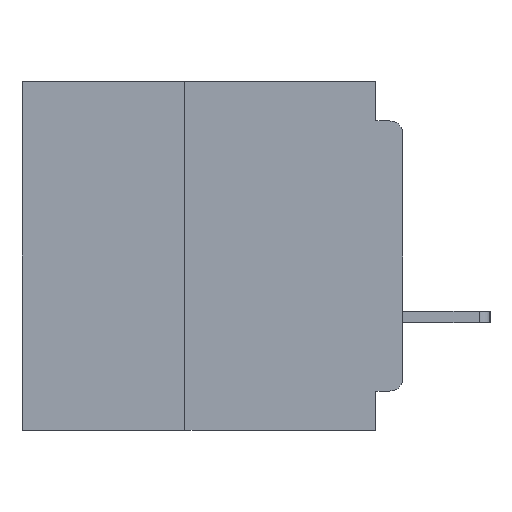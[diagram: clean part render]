
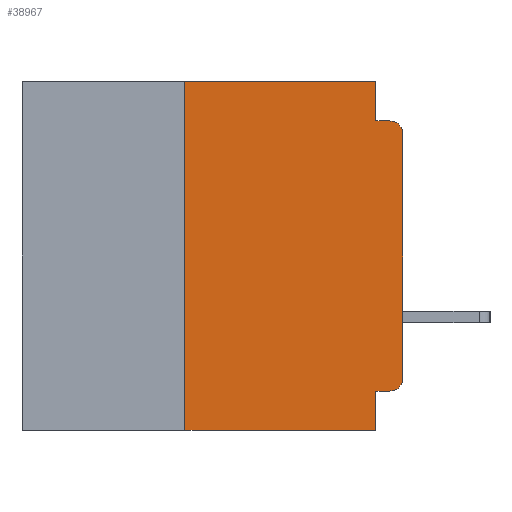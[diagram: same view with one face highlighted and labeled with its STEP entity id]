
A CAD part, left-side view. The second image highlights one B-rep face of the part: STEP entity #38967.
In plain terms, the highlighted planar face has unit normal (-1, 0, 0).
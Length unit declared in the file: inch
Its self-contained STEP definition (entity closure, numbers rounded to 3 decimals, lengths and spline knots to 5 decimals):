
#1255 = VERTEX_POINT ( 'NONE', #56523 ) ;
#1685 = EDGE_CURVE ( 'NONE', #65093, #3620, #50024, .T. ) ;
#2430 = CARTESIAN_POINT ( 'NONE',  ( 0., 0.015, -0.355 ) ) ;
#2866 = VECTOR ( 'NONE', #17412, 39.37008 ) ;
#3620 = VERTEX_POINT ( 'NONE', #35172 ) ;
#4160 = PLANE ( 'NONE',  #16183 ) ;
#7343 = CARTESIAN_POINT ( 'NONE',  ( 0., 0.031, 0. ) ) ;
#7485 = CARTESIAN_POINT ( 'NONE',  ( 0., 0.015, -0.34 ) ) ;
#7657 = LINE ( 'NONE', #48281, #29862 ) ;
#7855 = DIRECTION ( 'NONE',  ( 0., 0., 1. ) ) ;
#8508 = EDGE_CURVE ( 'NONE', #1255, #65093, #61952, .T. ) ;
#9325 = ORIENTED_EDGE ( 'NONE', *, *, #62804, .F. ) ;
#10684 = EDGE_LOOP ( 'NONE', ( #64152, #30747, #50176, #18854, #46270, #9325, #41486, #35100, #15360, #61409 ) ) ;
#12639 = DIRECTION ( 'NONE',  ( 0., 0., -1. ) ) ;
#14378 = DIRECTION ( 'NONE',  ( 1., 0., 0. ) ) ;
#14414 = VECTOR ( 'NONE', #64098, 39.37008 ) ;
#15226 = VECTOR ( 'NONE', #37704, 39.37008 ) ;
#15360 = ORIENTED_EDGE ( 'NONE', *, *, #49907, .F. ) ;
#16049 = EDGE_CURVE ( 'NONE', #16051, #1255, #30943, .T. ) ;
#16051 = VERTEX_POINT ( 'NONE', #2430 ) ;
#16183 = AXIS2_PLACEMENT_3D ( 'NONE', #34315, #14378, #49643 ) ;
#16608 = CARTESIAN_POINT ( 'NONE',  ( 0., 0., 0. ) ) ;
#16840 = LINE ( 'NONE', #7343, #15226 ) ;
#17412 = DIRECTION ( 'NONE',  ( 0., 0., -1. ) ) ;
#18854 = ORIENTED_EDGE ( 'NONE', *, *, #26511, .F. ) ;
#20239 = VECTOR ( 'NONE', #26630, 39.37008 ) ;
#20734 = DIRECTION ( 'NONE',  ( 0., -1., 0. ) ) ;
#21391 = EDGE_CURVE ( 'NONE', #46968, #26798, #23236, .T. ) ;
#21931 = AXIS2_PLACEMENT_3D ( 'NONE', #43266, #43131, #43058 ) ;
#23236 = LINE ( 'NONE', #50883, #36675 ) ;
#25878 = CARTESIAN_POINT ( 'NONE',  ( 0., 0.25, 0. ) ) ;
#26257 = VECTOR ( 'NONE', #27592, 39.37008 ) ;
#26511 = EDGE_CURVE ( 'NONE', #58493, #40507, #16840, .T. ) ;
#26630 = DIRECTION ( 'NONE',  ( 0., -1., 0. ) ) ;
#26798 = VERTEX_POINT ( 'NONE', #64729 ) ;
#27592 = DIRECTION ( 'NONE',  ( 0., 1., 0. ) ) ;
#27931 = LINE ( 'NONE', #29056, #14414 ) ;
#29056 = CARTESIAN_POINT ( 'NONE',  ( 0., 0., -0.045 ) ) ;
#29128 = VERTEX_POINT ( 'NONE', #36117 ) ;
#29835 = LINE ( 'NONE', #47358, #2866 ) ;
#29862 = VECTOR ( 'NONE', #7855, 39.37008 ) ;
#30747 = ORIENTED_EDGE ( 'NONE', *, *, #1685, .T. ) ;
#30943 = CIRCLE ( 'NONE', #55826, 0.015 ) ;
#31742 = CARTESIAN_POINT ( 'NONE',  ( 0., 0.437, 0. ) ) ;
#32212 = VECTOR ( 'NONE', #41752, 39.37008 ) ;
#33148 = CARTESIAN_POINT ( 'NONE',  ( 0., 0.25, -0.4 ) ) ;
#34315 = CARTESIAN_POINT ( 'NONE',  ( 0., 0.437, 0. ) ) ;
#35100 = ORIENTED_EDGE ( 'NONE', *, *, #44341, .F. ) ;
#35172 = CARTESIAN_POINT ( 'NONE',  ( 0., 0.015, -0.045 ) ) ;
#35285 = LINE ( 'NONE', #31742, #20239 ) ;
#36117 = CARTESIAN_POINT ( 'NONE',  ( 0., 0.031, -0.355 ) ) ;
#36675 = VECTOR ( 'NONE', #20734, 39.37008 ) ;
#37704 = DIRECTION ( 'NONE',  ( 0., 0., -1. ) ) ;
#38109 = CARTESIAN_POINT ( 'NONE',  ( 0., 0.031, -0.045 ) ) ;
#38646 = EDGE_CURVE ( 'NONE', #43870, #58493, #35285, .T. ) ;
#38967 = ADVANCED_FACE ( 'NONE', ( #41519 ), #4160, .F. ) ;
#39283 = CARTESIAN_POINT ( 'NONE',  ( 0., 0.031, 0. ) ) ;
#40507 = VERTEX_POINT ( 'NONE', #38109 ) ;
#41486 = ORIENTED_EDGE ( 'NONE', *, *, #21391, .T. ) ;
#41519 = FACE_OUTER_BOUND ( 'NONE', #10684, .T. ) ;
#41752 = DIRECTION ( 'NONE',  ( 0., 0., 1. ) ) ;
#42884 = DIRECTION ( 'NONE',  ( -1., 0., 0. ) ) ;
#43058 = DIRECTION ( 'NONE',  ( 0., 0., -1. ) ) ;
#43131 = DIRECTION ( 'NONE',  ( -1., 0., 0. ) ) ;
#43182 = CARTESIAN_POINT ( 'NONE',  ( 0., 0., -0.06 ) ) ;
#43266 = CARTESIAN_POINT ( 'NONE',  ( 0., 0.015, -0.06 ) ) ;
#43870 = VERTEX_POINT ( 'NONE', #25878 ) ;
#44341 = EDGE_CURVE ( 'NONE', #29128, #26798, #29835, .T. ) ;
#46270 = ORIENTED_EDGE ( 'NONE', *, *, #38646, .F. ) ;
#46968 = VERTEX_POINT ( 'NONE', #33148 ) ;
#47358 = CARTESIAN_POINT ( 'NONE',  ( 0., 0.031, -0.4 ) ) ;
#48281 = CARTESIAN_POINT ( 'NONE',  ( 0., 0.25, -0.4 ) ) ;
#49486 = EDGE_CURVE ( 'NONE', #40507, #3620, #27931, .T. ) ;
#49643 = DIRECTION ( 'NONE',  ( 0., 0., -1. ) ) ;
#49907 = EDGE_CURVE ( 'NONE', #16051, #29128, #54577, .T. ) ;
#50024 = CIRCLE ( 'NONE', #21931, 0.015 ) ;
#50176 = ORIENTED_EDGE ( 'NONE', *, *, #49486, .F. ) ;
#50883 = CARTESIAN_POINT ( 'NONE',  ( 0., 0.437, -0.4 ) ) ;
#52625 = CARTESIAN_POINT ( 'NONE',  ( 0., 0., -0.355 ) ) ;
#54577 = LINE ( 'NONE', #52625, #26257 ) ;
#55826 = AXIS2_PLACEMENT_3D ( 'NONE', #7485, #42884, #12639 ) ;
#56523 = CARTESIAN_POINT ( 'NONE',  ( 0., 0., -0.34 ) ) ;
#58493 = VERTEX_POINT ( 'NONE', #39283 ) ;
#61409 = ORIENTED_EDGE ( 'NONE', *, *, #16049, .T. ) ;
#61952 = LINE ( 'NONE', #16608, #32212 ) ;
#62804 = EDGE_CURVE ( 'NONE', #46968, #43870, #7657, .T. ) ;
#64098 = DIRECTION ( 'NONE',  ( 0., -1., 0. ) ) ;
#64152 = ORIENTED_EDGE ( 'NONE', *, *, #8508, .T. ) ;
#64729 = CARTESIAN_POINT ( 'NONE',  ( 0., 0.031, -0.4 ) ) ;
#65093 = VERTEX_POINT ( 'NONE', #43182 ) ;
